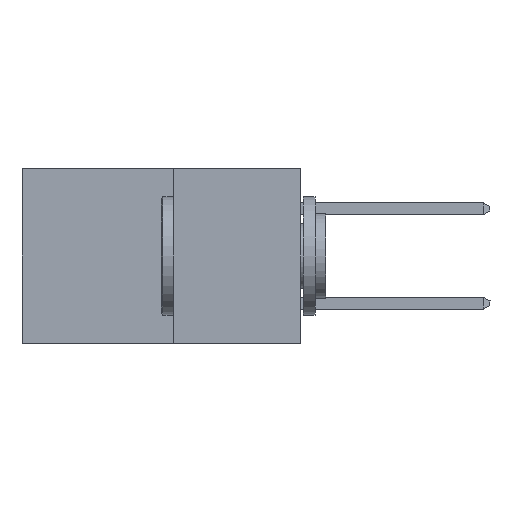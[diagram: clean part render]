
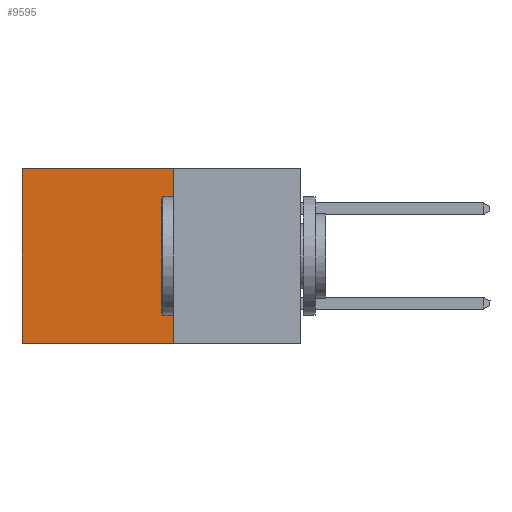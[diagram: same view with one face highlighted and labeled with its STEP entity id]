
A CAD part, left-side view. The second image highlights one B-rep face of the part: STEP entity #9595.
In plain terms, the highlighted planar face has unit normal (-1, 0, 0).
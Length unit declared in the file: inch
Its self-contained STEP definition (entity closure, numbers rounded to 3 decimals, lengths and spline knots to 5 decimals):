
#421 = CARTESIAN_POINT ( 'NONE',  ( 0.277, 0.59, -0.37 ) ) ;
#474 = VECTOR ( 'NONE', #6976, 39.37008 ) ;
#727 = LINE ( 'NONE', #10603, #5221 ) ;
#801 = VERTEX_POINT ( 'NONE', #421 ) ;
#909 = CARTESIAN_POINT ( 'NONE',  ( 0.277, 0.27, -0.37 ) ) ;
#1155 = EDGE_CURVE ( 'NONE', #6389, #801, #727, .T. ) ;
#1264 = EDGE_CURVE ( 'NONE', #10283, #6389, #5897, .T. ) ;
#1870 = DIRECTION ( 'NONE',  ( 1., 0., 0. ) ) ;
#4002 = VERTEX_POINT ( 'NONE', #10773 ) ;
#4440 = EDGE_CURVE ( 'NONE', #4002, #801, #7895, .T. ) ;
#4751 = CARTESIAN_POINT ( 'NONE',  ( 0.277, 0.27, -0.37 ) ) ;
#4804 = DIRECTION ( 'NONE',  ( 0., 1., 0. ) ) ;
#5221 = VECTOR ( 'NONE', #8472, 39.37008 ) ;
#5428 = CARTESIAN_POINT ( 'NONE',  ( 0.277, 0.27, 0. ) ) ;
#5442 = EDGE_CURVE ( 'NONE', #10283, #4002, #9555, .T. ) ;
#5809 = ORIENTED_EDGE ( 'NONE', *, *, #1155, .T. ) ;
#5897 = LINE ( 'NONE', #5428, #9893 ) ;
#6122 = ORIENTED_EDGE ( 'NONE', *, *, #4440, .F. ) ;
#6255 = PLANE ( 'NONE',  #7910 ) ;
#6389 = VERTEX_POINT ( 'NONE', #9537 ) ;
#6976 = DIRECTION ( 'NONE',  ( 0., 0., -1. ) ) ;
#7026 = CARTESIAN_POINT ( 'NONE',  ( 0.277, 0.27, -0.37 ) ) ;
#7099 = DIRECTION ( 'NONE',  ( 0., 1., 0. ) ) ;
#7294 = ORIENTED_EDGE ( 'NONE', *, *, #5442, .F. ) ;
#7882 = DIRECTION ( 'NONE',  ( 0., 0., -1. ) ) ;
#7895 = LINE ( 'NONE', #4751, #9946 ) ;
#7910 = AXIS2_PLACEMENT_3D ( 'NONE', #909, #1870, #7882 ) ;
#8264 = ORIENTED_EDGE ( 'NONE', *, *, #1264, .T. ) ;
#8472 = DIRECTION ( 'NONE',  ( 0., 0., -1. ) ) ;
#8615 = CARTESIAN_POINT ( 'NONE',  ( 0.277, 0.27, 0. ) ) ;
#9537 = CARTESIAN_POINT ( 'NONE',  ( 0.277, 0.59, 0. ) ) ;
#9555 = LINE ( 'NONE', #7026, #474 ) ;
#9595 = ADVANCED_FACE ( 'NONE', ( #9611 ), #6255, .F. ) ;
#9611 = FACE_OUTER_BOUND ( 'NONE', #10701, .T. ) ;
#9893 = VECTOR ( 'NONE', #7099, 39.37008 ) ;
#9946 = VECTOR ( 'NONE', #4804, 39.37008 ) ;
#10283 = VERTEX_POINT ( 'NONE', #8615 ) ;
#10603 = CARTESIAN_POINT ( 'NONE',  ( 0.277, 0.59, -0.37 ) ) ;
#10701 = EDGE_LOOP ( 'NONE', ( #5809, #6122, #7294, #8264 ) ) ;
#10773 = CARTESIAN_POINT ( 'NONE',  ( 0.277, 0.27, -0.37 ) ) ;
